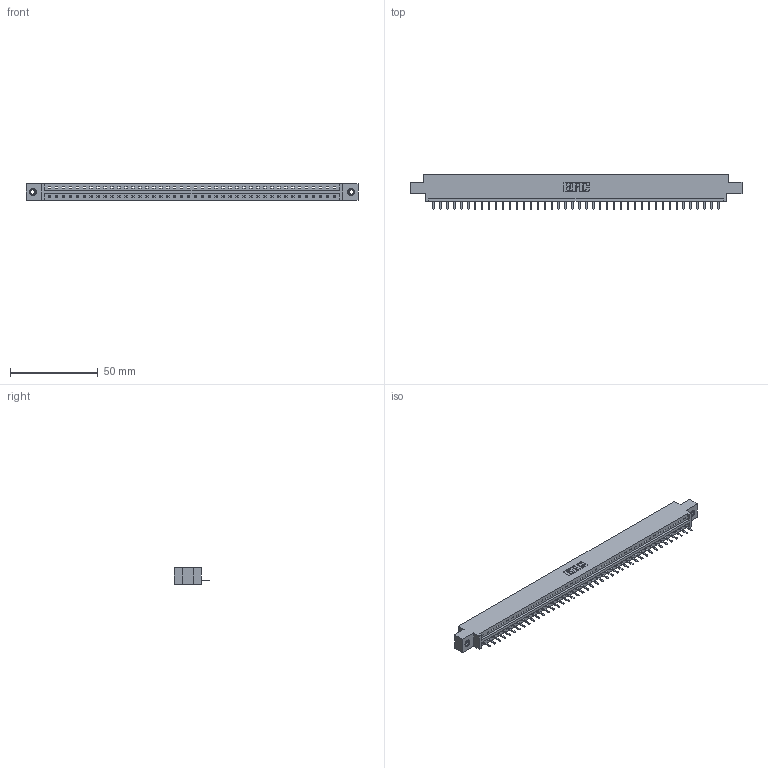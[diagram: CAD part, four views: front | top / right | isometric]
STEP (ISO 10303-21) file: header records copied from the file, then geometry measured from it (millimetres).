
FILE_DESCRIPTION (( 'STEP AP203' ), '1' );
FILE_NAME ('337-042-520-607.STEP', '2019-10-01T21:40:33', ( '' ), ( '' ), 'SwSTEP 2.0', 'SolidWorks 2016', '' );
FILE_SCHEMA (( 'CONFIG_CONTROL_DESIGN' ));
Length unit declared in the file: inch
Products named in the file (4): 345-250-001_345-250-005-103; 337-042-520-607; 337 Part_0.170 Offset - 0.156 Dia-TI; 345-292-001_345-293-120
Assembly tree (45 placements, depth 2):
  337-042-520-607
    337 Part_0.170 Offset - 0.156 Dia-TI
    345-292-001_345-293-120  x42
    345-250-001_345-250-005-103  x2
Bounding box: 189.43 x 20.02 x 9.4 mm (x, y, z)
Volume: 19436.6 mm3; surface area: 19787.4 mm2
Topology: 45 solids, 45 shells, 2950 faces, 8691 edges, 5674 vertices
Faces by surface type: plane 2122, cylinder 812, cone 12, torus 4
Entity records: 32652 total; most frequent: CARTESIAN_POINT 5679, ORIENTED_EDGE 5638, DIRECTION 4801, EDGE_CURVE 2819, VECTOR 2667, LINE 2667, VERTEX_POINT 1872, AXIS2_PLACEMENT_3D 1067
